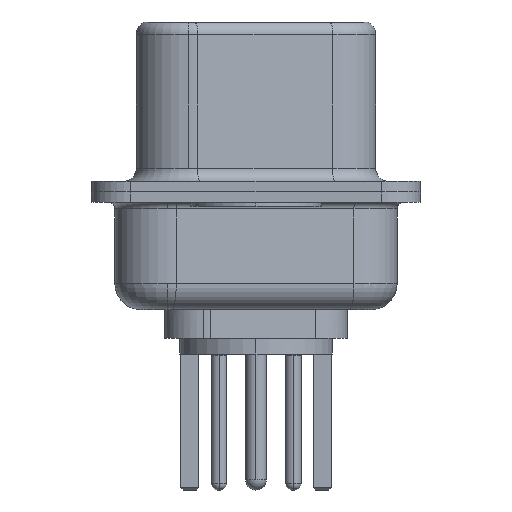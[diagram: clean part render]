
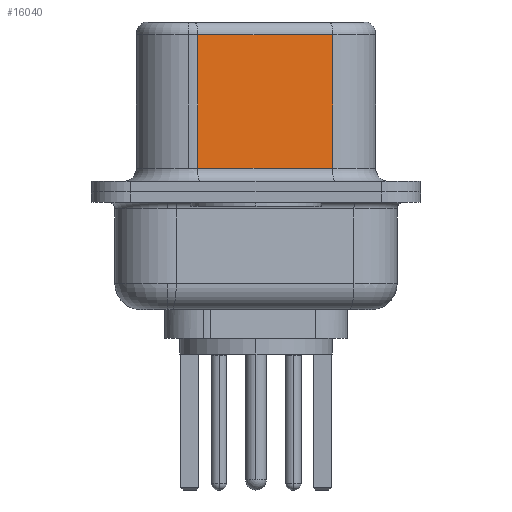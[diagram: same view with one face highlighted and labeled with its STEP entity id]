
A CAD part, left-side view. The second image highlights one B-rep face of the part: STEP entity #16040.
In plain terms, the highlighted planar face has unit normal (-0.985, -0.174, 0).
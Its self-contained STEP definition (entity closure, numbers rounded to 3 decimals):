
#152 = EDGE_CURVE ( 'NONE', #7977, #15237, #2992, .T. ) ;
#208 = EDGE_CURVE ( 'NONE', #7977, #2920, #4946, .T. ) ;
#692 = ORIENTED_EDGE ( 'NONE', *, *, #152, .F. ) ;
#941 = ORIENTED_EDGE ( 'NONE', *, *, #208, .T. ) ;
#1844 = EDGE_LOOP ( 'NONE', ( #692, #941, #15190, #7090 ) ) ;
#2396 = DIRECTION ( 'NONE',  ( 0., 0., -1. ) ) ;
#2920 = VERTEX_POINT ( 'NONE', #15073 ) ;
#2992 = LINE ( 'NONE', #12129, #16368 ) ;
#3057 = LINE ( 'NONE', #5906, #9996 ) ;
#3286 = EDGE_CURVE ( 'NONE', #2920, #17092, #13238, .T. ) ;
#3428 = CARTESIAN_POINT ( 'NONE',  ( 4.585, -2.927, 0.9 ) ) ;
#4946 = LINE ( 'NONE', #10928, #11861 ) ;
#5320 = DIRECTION ( 'NONE',  ( 0.985, 0.174, 0. ) ) ;
#5906 = CARTESIAN_POINT ( 'NONE',  ( 4.585, -2.927, 0.9 ) ) ;
#6015 = AXIS2_PLACEMENT_3D ( 'NONE', #17704, #5320, #14965 ) ;
#7090 = ORIENTED_EDGE ( 'NONE', *, *, #10376, .T. ) ;
#7479 = CARTESIAN_POINT ( 'NONE',  ( 4.585, -2.927, 6.02 ) ) ;
#7977 = VERTEX_POINT ( 'NONE', #7479 ) ;
#9996 = VECTOR ( 'NONE', #15560, 1000. ) ;
#10376 = EDGE_CURVE ( 'NONE', #17092, #15237, #3057, .T. ) ;
#10833 = PLANE ( 'NONE',  #6015 ) ;
#10928 = CARTESIAN_POINT ( 'NONE',  ( 4.585, -2.927, 6.02 ) ) ;
#10985 = DIRECTION ( 'NONE',  ( -0.174, 0.985, 0. ) ) ;
#11861 = VECTOR ( 'NONE', #10985, 1000. ) ;
#12007 = DIRECTION ( 'NONE',  ( 0., 0., -1. ) ) ;
#12129 = CARTESIAN_POINT ( 'NONE',  ( 4.585, -2.927, 6.52 ) ) ;
#13238 = LINE ( 'NONE', #13717, #13653 ) ;
#13258 = FACE_OUTER_BOUND ( 'NONE', #1844, .T. ) ;
#13653 = VECTOR ( 'NONE', #2396, 1000. ) ;
#13717 = CARTESIAN_POINT ( 'NONE',  ( 3.675, 2.233, 6.52 ) ) ;
#14965 = DIRECTION ( 'NONE',  ( -0.174, 0.985, 0. ) ) ;
#15073 = CARTESIAN_POINT ( 'NONE',  ( 3.675, 2.233, 6.02 ) ) ;
#15190 = ORIENTED_EDGE ( 'NONE', *, *, #3286, .T. ) ;
#15237 = VERTEX_POINT ( 'NONE', #3428 ) ;
#15560 = DIRECTION ( 'NONE',  ( 0.174, -0.985, 0. ) ) ;
#16040 = ADVANCED_FACE ( 'NONE', ( #13258 ), #10833, .F. ) ;
#16368 = VECTOR ( 'NONE', #12007, 1000. ) ;
#17092 = VERTEX_POINT ( 'NONE', #17191 ) ;
#17191 = CARTESIAN_POINT ( 'NONE',  ( 3.675, 2.233, 0.9 ) ) ;
#17704 = CARTESIAN_POINT ( 'NONE',  ( 4.585, -2.927, 6.52 ) ) ;
